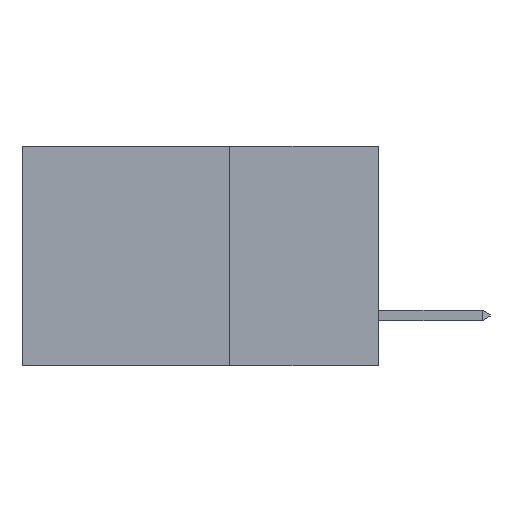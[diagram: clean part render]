
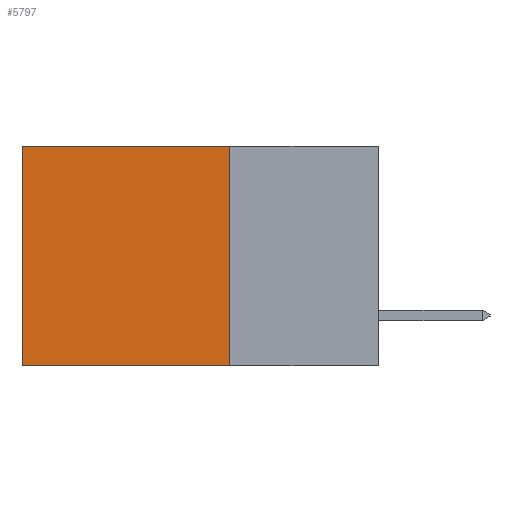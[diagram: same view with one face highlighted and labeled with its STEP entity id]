
A CAD part, left-side view. The second image highlights one B-rep face of the part: STEP entity #5797.
In plain terms, the highlighted planar face has unit normal (-1, 0, 0).
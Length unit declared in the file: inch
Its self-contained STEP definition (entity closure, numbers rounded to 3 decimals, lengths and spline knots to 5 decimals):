
#66 = CARTESIAN_POINT ( 'NONE',  ( 0.2615, 0.6, 0. ) ) ;
#358 = LINE ( 'NONE', #4751, #2128 ) ;
#708 = CARTESIAN_POINT ( 'NONE',  ( 0.2615, 0.25, 0. ) ) ;
#992 = LINE ( 'NONE', #1545, #2985 ) ;
#1442 = CARTESIAN_POINT ( 'NONE',  ( 0.2615, 0.25, -0.37 ) ) ;
#1545 = CARTESIAN_POINT ( 'NONE',  ( 0.2615, 0.25, -0.37 ) ) ;
#1757 = CARTESIAN_POINT ( 'NONE',  ( 0.2615, 0.6, -0.37 ) ) ;
#1974 = CARTESIAN_POINT ( 'NONE',  ( 0.2615, 0.25, -0.37 ) ) ;
#2128 = VECTOR ( 'NONE', #4778, 39.37008 ) ;
#2230 = ORIENTED_EDGE ( 'NONE', *, *, #8956, .F. ) ;
#2302 = DIRECTION ( 'NONE',  ( 0., 1., 0. ) ) ;
#2464 = VERTEX_POINT ( 'NONE', #6157 ) ;
#2864 = VERTEX_POINT ( 'NONE', #1442 ) ;
#2985 = VECTOR ( 'NONE', #2302, 39.37008 ) ;
#3611 = CARTESIAN_POINT ( 'NONE',  ( 0.2615, 0.25, -0.37 ) ) ;
#4077 = EDGE_CURVE ( 'NONE', #5432, #4720, #358, .T. ) ;
#4231 = DIRECTION ( 'NONE',  ( 0., 0., -1. ) ) ;
#4351 = DIRECTION ( 'NONE',  ( 1., 0., 0. ) ) ;
#4480 = ORIENTED_EDGE ( 'NONE', *, *, #4077, .T. ) ;
#4492 = DIRECTION ( 'NONE',  ( 0., 1., 0. ) ) ;
#4720 = VERTEX_POINT ( 'NONE', #1757 ) ;
#4751 = CARTESIAN_POINT ( 'NONE',  ( 0.2615, 0.6, -0.37 ) ) ;
#4778 = DIRECTION ( 'NONE',  ( 0., 0., -1. ) ) ;
#5432 = VERTEX_POINT ( 'NONE', #66 ) ;
#5797 = ADVANCED_FACE ( 'NONE', ( #9170 ), #8048, .F. ) ;
#6157 = CARTESIAN_POINT ( 'NONE',  ( 0.2615, 0.25, 0. ) ) ;
#6158 = LINE ( 'NONE', #1974, #7888 ) ;
#6590 = ORIENTED_EDGE ( 'NONE', *, *, #7017, .F. ) ;
#6867 = EDGE_LOOP ( 'NONE', ( #4480, #2230, #6590, #7190 ) ) ;
#6969 = VECTOR ( 'NONE', #4492, 39.37008 ) ;
#7017 = EDGE_CURVE ( 'NONE', #2464, #2864, #6158, .T. ) ;
#7190 = ORIENTED_EDGE ( 'NONE', *, *, #8909, .T. ) ;
#7888 = VECTOR ( 'NONE', #4231, 39.37008 ) ;
#8048 = PLANE ( 'NONE',  #9321 ) ;
#8903 = LINE ( 'NONE', #708, #6969 ) ;
#8909 = EDGE_CURVE ( 'NONE', #2464, #5432, #8903, .T. ) ;
#8956 = EDGE_CURVE ( 'NONE', #2864, #4720, #992, .T. ) ;
#9170 = FACE_OUTER_BOUND ( 'NONE', #6867, .T. ) ;
#9321 = AXIS2_PLACEMENT_3D ( 'NONE', #3611, #4351, #9521 ) ;
#9521 = DIRECTION ( 'NONE',  ( 0., 0., -1. ) ) ;
